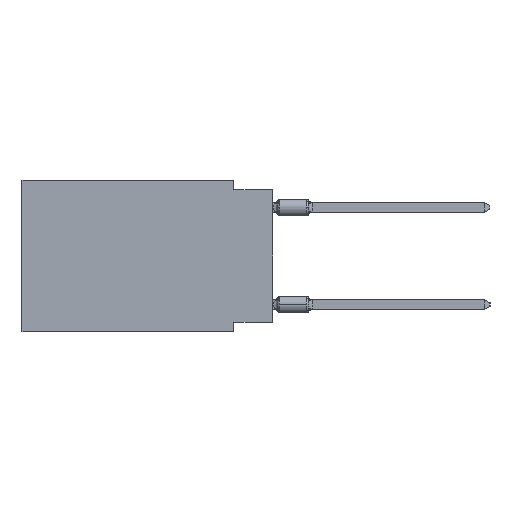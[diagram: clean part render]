
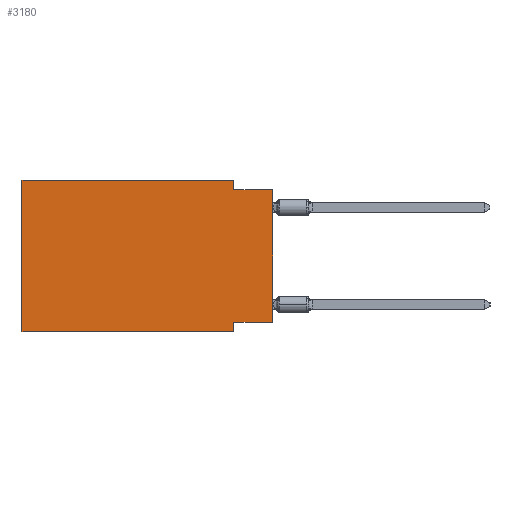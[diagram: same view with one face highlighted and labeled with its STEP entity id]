
A CAD part, left-side view. The second image highlights one B-rep face of the part: STEP entity #3180.
In plain terms, the highlighted planar face has unit normal (-1, 0, 0).
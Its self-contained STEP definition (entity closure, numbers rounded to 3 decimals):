
#339 = CARTESIAN_POINT ( 'NONE',  ( 0., 2.54, -9.906 ) ) ;
#711 = VERTEX_POINT ( 'NONE', #3215 ) ;
#996 = EDGE_CURVE ( 'NONE', #29804, #711, #6404, .T. ) ;
#1401 = ORIENTED_EDGE ( 'NONE', *, *, #39059, .F. ) ;
#2199 = ORIENTED_EDGE ( 'NONE', *, *, #996, .F. ) ;
#2424 = VECTOR ( 'NONE', #14201, 1000. ) ;
#2684 = DIRECTION ( 'NONE',  ( 0., 0., -1. ) ) ;
#2940 = LINE ( 'NONE', #33194, #2424 ) ;
#3180 = ADVANCED_FACE ( 'NONE', ( #29536 ), #41267, .F. ) ;
#3215 = CARTESIAN_POINT ( 'NONE',  ( 0., 2.54, -0.635 ) ) ;
#3640 = CARTESIAN_POINT ( 'NONE',  ( 0., 2.54, 0. ) ) ;
#4871 = CARTESIAN_POINT ( 'NONE',  ( 0., 2.54, -9.906 ) ) ;
#6404 = LINE ( 'NONE', #43897, #48621 ) ;
#7189 = VERTEX_POINT ( 'NONE', #4871 ) ;
#8241 = CARTESIAN_POINT ( 'NONE',  ( 0., 0., -9.271 ) ) ;
#8925 = LINE ( 'NONE', #44139, #29109 ) ;
#9893 = DIRECTION ( 'NONE',  ( 0., 0., 1. ) ) ;
#13803 = EDGE_CURVE ( 'NONE', #47412, #7189, #33554, .T. ) ;
#13969 = CARTESIAN_POINT ( 'NONE',  ( 0., 2.54, -9.271 ) ) ;
#14201 = DIRECTION ( 'NONE',  ( 0., -1., 0. ) ) ;
#14616 = CARTESIAN_POINT ( 'NONE',  ( 0., 16.383, 0. ) ) ;
#15352 = CARTESIAN_POINT ( 'NONE',  ( 0., 16.383, -9.906 ) ) ;
#17455 = DIRECTION ( 'NONE',  ( 0., -1., 0. ) ) ;
#17539 = VECTOR ( 'NONE', #44537, 1000. ) ;
#18503 = EDGE_CURVE ( 'NONE', #47412, #29067, #48850, .T. ) ;
#18738 = ORIENTED_EDGE ( 'NONE', *, *, #46620, .F. ) ;
#19328 = ORIENTED_EDGE ( 'NONE', *, *, #18503, .F. ) ;
#19753 = VECTOR ( 'NONE', #17455, 1000. ) ;
#20798 = EDGE_CURVE ( 'NONE', #29067, #29804, #2940, .T. ) ;
#20963 = ORIENTED_EDGE ( 'NONE', *, *, #20798, .F. ) ;
#21071 = EDGE_CURVE ( 'NONE', #46474, #44193, #8925, .T. ) ;
#21947 = CARTESIAN_POINT ( 'NONE',  ( 0., 0., -9.271 ) ) ;
#22090 = AXIS2_PLACEMENT_3D ( 'NONE', #34926, #48783, #44796 ) ;
#23849 = VERTEX_POINT ( 'NONE', #13969 ) ;
#27878 = VECTOR ( 'NONE', #2684, 1000. ) ;
#29067 = VERTEX_POINT ( 'NONE', #33465 ) ;
#29109 = VECTOR ( 'NONE', #9893, 1000. ) ;
#29181 = DIRECTION ( 'NONE',  ( 0., 1., 0. ) ) ;
#29319 = ORIENTED_EDGE ( 'NONE', *, *, #13803, .T. ) ;
#29536 = FACE_OUTER_BOUND ( 'NONE', #38428, .T. ) ;
#29552 = CARTESIAN_POINT ( 'NONE',  ( 0., 16.383, -9.906 ) ) ;
#29804 = VERTEX_POINT ( 'NONE', #3640 ) ;
#29844 = DIRECTION ( 'NONE',  ( 0., 0., 1. ) ) ;
#30574 = ORIENTED_EDGE ( 'NONE', *, *, #21071, .T. ) ;
#31989 = CARTESIAN_POINT ( 'NONE',  ( 0., 0., -0.635 ) ) ;
#33194 = CARTESIAN_POINT ( 'NONE',  ( 0., 16.383, 0. ) ) ;
#33465 = CARTESIAN_POINT ( 'NONE',  ( 0., 16.383, 0. ) ) ;
#33554 = LINE ( 'NONE', #29552, #17539 ) ;
#34926 = CARTESIAN_POINT ( 'NONE',  ( 0., 16.383, 0. ) ) ;
#36161 = DIRECTION ( 'NONE',  ( 0., 0., -1. ) ) ;
#37572 = VECTOR ( 'NONE', #29181, 1000. ) ;
#38428 = EDGE_LOOP ( 'NONE', ( #30574, #18738, #2199, #20963, #19328, #29319, #1401, #38982 ) ) ;
#38982 = ORIENTED_EDGE ( 'NONE', *, *, #42101, .F. ) ;
#39059 = EDGE_CURVE ( 'NONE', #23849, #7189, #48665, .T. ) ;
#39887 = CARTESIAN_POINT ( 'NONE',  ( 0., 0., -0.635 ) ) ;
#41267 = PLANE ( 'NONE',  #22090 ) ;
#42101 = EDGE_CURVE ( 'NONE', #46474, #23849, #44692, .T. ) ;
#43710 = LINE ( 'NONE', #31989, #19753 ) ;
#43897 = CARTESIAN_POINT ( 'NONE',  ( 0., 2.54, 0. ) ) ;
#44139 = CARTESIAN_POINT ( 'NONE',  ( 0., 0., 0. ) ) ;
#44193 = VERTEX_POINT ( 'NONE', #39887 ) ;
#44537 = DIRECTION ( 'NONE',  ( 0., -1., 0. ) ) ;
#44692 = LINE ( 'NONE', #21947, #37572 ) ;
#44796 = DIRECTION ( 'NONE',  ( 0., 0., -1. ) ) ;
#46474 = VERTEX_POINT ( 'NONE', #8241 ) ;
#46620 = EDGE_CURVE ( 'NONE', #711, #44193, #43710, .T. ) ;
#47099 = VECTOR ( 'NONE', #29844, 1000. ) ;
#47412 = VERTEX_POINT ( 'NONE', #15352 ) ;
#48621 = VECTOR ( 'NONE', #36161, 1000. ) ;
#48665 = LINE ( 'NONE', #339, #27878 ) ;
#48783 = DIRECTION ( 'NONE',  ( 1., 0., 0. ) ) ;
#48850 = LINE ( 'NONE', #14616, #47099 ) ;
